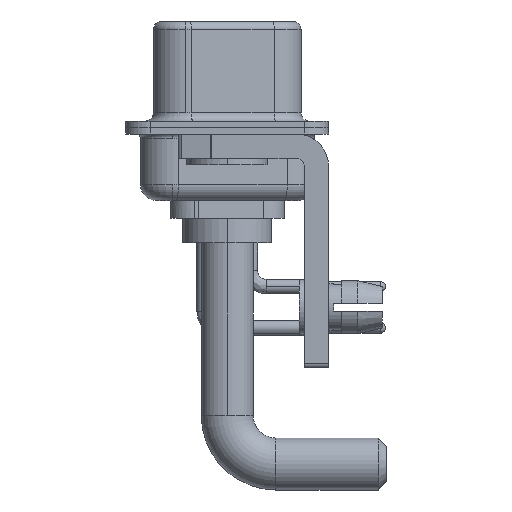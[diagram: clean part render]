
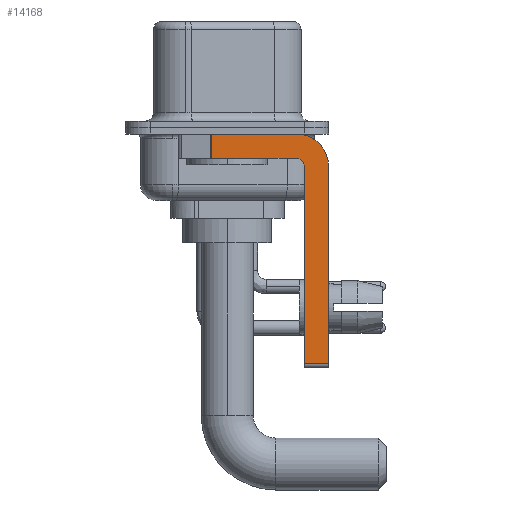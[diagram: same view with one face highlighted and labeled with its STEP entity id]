
A CAD part, left-side view. The second image highlights one B-rep face of the part: STEP entity #14168.
In plain terms, the highlighted planar face has unit normal (-1, 0, 0).
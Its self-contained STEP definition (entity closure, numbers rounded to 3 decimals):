
#398 = VERTEX_POINT ( 'NONE', #3564 ) ;
#563 = VERTEX_POINT ( 'NONE', #5437 ) ;
#916 = VERTEX_POINT ( 'NONE', #23170 ) ;
#1753 = DIRECTION ( 'NONE',  ( 0., 0., -1. ) ) ;
#1857 = LINE ( 'NONE', #25666, #8241 ) ;
#1941 = ORIENTED_EDGE ( 'NONE', *, *, #12348, .F. ) ;
#2040 = DIRECTION ( 'NONE',  ( 0., 0., -1. ) ) ;
#2108 = CARTESIAN_POINT ( 'NONE',  ( -2.9, 0.978, -0.4 ) ) ;
#2377 = CARTESIAN_POINT ( 'NONE',  ( -2.9, -4.25, -2.4 ) ) ;
#2700 = ORIENTED_EDGE ( 'NONE', *, *, #9744, .T. ) ;
#3564 = CARTESIAN_POINT ( 'NONE',  ( -2.9, -4.25, -0.4 ) ) ;
#3682 = VECTOR ( 'NONE', #14095, 1000. ) ;
#3843 = ORIENTED_EDGE ( 'NONE', *, *, #18338, .F. ) ;
#4151 = AXIS2_PLACEMENT_3D ( 'NONE', #17599, #23833, #17059 ) ;
#4231 = DIRECTION ( 'NONE',  ( 1., 0., 0. ) ) ;
#5195 = EDGE_LOOP ( 'NONE', ( #20645, #2700, #12377, #22074, #3843, #8098, #1941, #6665 ) ) ;
#5309 = LINE ( 'NONE', #27131, #6953 ) ;
#5437 = CARTESIAN_POINT ( 'NONE',  ( -2.9, -4.25, -1.9 ) ) ;
#5597 = VERTEX_POINT ( 'NONE', #2108 ) ;
#6665 = ORIENTED_EDGE ( 'NONE', *, *, #10041, .F. ) ;
#6683 = DIRECTION ( 'NONE',  ( 0., 0., 1. ) ) ;
#6825 = AXIS2_PLACEMENT_3D ( 'NONE', #14381, #25133, #1753 ) ;
#6953 = VECTOR ( 'NONE', #16519, 1000. ) ;
#8098 = ORIENTED_EDGE ( 'NONE', *, *, #23374, .T. ) ;
#8161 = VERTEX_POINT ( 'NONE', #24841 ) ;
#8241 = VECTOR ( 'NONE', #10519, 1000. ) ;
#9744 = EDGE_CURVE ( 'NONE', #5597, #19030, #25699, .T. ) ;
#9855 = LINE ( 'NONE', #25408, #3682 ) ;
#9945 = DIRECTION ( 'NONE',  ( 0., -1., 0. ) ) ;
#10041 = EDGE_CURVE ( 'NONE', #398, #13597, #19855, .T. ) ;
#10075 = LINE ( 'NONE', #18722, #22413 ) ;
#10519 = DIRECTION ( 'NONE',  ( 0., -1., 0. ) ) ;
#10530 = CARTESIAN_POINT ( 'NONE',  ( -2.9, -4.75, -14.8 ) ) ;
#10806 = VECTOR ( 'NONE', #2040, 1000. ) ;
#12035 = CARTESIAN_POINT ( 'NONE',  ( -2.9, -4.75, -2.4 ) ) ;
#12348 = EDGE_CURVE ( 'NONE', #13597, #916, #5309, .T. ) ;
#12377 = ORIENTED_EDGE ( 'NONE', *, *, #14148, .F. ) ;
#13597 = VERTEX_POINT ( 'NONE', #16269 ) ;
#14095 = DIRECTION ( 'NONE',  ( 0., 1., 0. ) ) ;
#14148 = EDGE_CURVE ( 'NONE', #563, #19030, #9855, .T. ) ;
#14168 = ADVANCED_FACE ( 'NONE', ( #18779 ), #16370, .F. ) ;
#14381 = CARTESIAN_POINT ( 'NONE',  ( -2.9, -4.25, -2.4 ) ) ;
#14436 = CARTESIAN_POINT ( 'NONE',  ( -2.9, 0.978, -1.9 ) ) ;
#14578 = CIRCLE ( 'NONE', #4151, 0.5 ) ;
#14879 = AXIS2_PLACEMENT_3D ( 'NONE', #2377, #4231, #19414 ) ;
#16269 = CARTESIAN_POINT ( 'NONE',  ( -2.9, -6.25, -2.4 ) ) ;
#16370 = PLANE ( 'NONE',  #6825 ) ;
#16519 = DIRECTION ( 'NONE',  ( 0., 0., -1. ) ) ;
#17059 = DIRECTION ( 'NONE',  ( 0., 0., 1. ) ) ;
#17599 = CARTESIAN_POINT ( 'NONE',  ( -2.9, -4.25, -2.4 ) ) ;
#18338 = EDGE_CURVE ( 'NONE', #8161, #27335, #21837, .T. ) ;
#18362 = EDGE_CURVE ( 'NONE', #27335, #563, #14578, .T. ) ;
#18722 = CARTESIAN_POINT ( 'NONE',  ( -2.9, -4.25, -14.55 ) ) ;
#18779 = FACE_OUTER_BOUND ( 'NONE', #5195, .T. ) ;
#19030 = VERTEX_POINT ( 'NONE', #14436 ) ;
#19414 = DIRECTION ( 'NONE',  ( 0., 0., -1. ) ) ;
#19855 = CIRCLE ( 'NONE', #14879, 2. ) ;
#20409 = EDGE_CURVE ( 'NONE', #5597, #398, #1857, .T. ) ;
#20645 = ORIENTED_EDGE ( 'NONE', *, *, #20409, .F. ) ;
#21837 = LINE ( 'NONE', #10530, #22693 ) ;
#22074 = ORIENTED_EDGE ( 'NONE', *, *, #18362, .F. ) ;
#22413 = VECTOR ( 'NONE', #9945, 1000. ) ;
#22693 = VECTOR ( 'NONE', #6683, 1000. ) ;
#23170 = CARTESIAN_POINT ( 'NONE',  ( -2.9, -6.25, -14.55 ) ) ;
#23374 = EDGE_CURVE ( 'NONE', #8161, #916, #10075, .T. ) ;
#23572 = CARTESIAN_POINT ( 'NONE',  ( -2.9, 0.978, -1.9 ) ) ;
#23833 = DIRECTION ( 'NONE',  ( -1., 0., 0. ) ) ;
#24841 = CARTESIAN_POINT ( 'NONE',  ( -2.9, -4.75, -14.55 ) ) ;
#25133 = DIRECTION ( 'NONE',  ( 1., 0., 0. ) ) ;
#25408 = CARTESIAN_POINT ( 'NONE',  ( -2.9, -4.25, -1.9 ) ) ;
#25666 = CARTESIAN_POINT ( 'NONE',  ( -2.9, 3., -0.4 ) ) ;
#25699 = LINE ( 'NONE', #23572, #10806 ) ;
#27131 = CARTESIAN_POINT ( 'NONE',  ( -2.9, -6.25, -2.4 ) ) ;
#27335 = VERTEX_POINT ( 'NONE', #12035 ) ;
